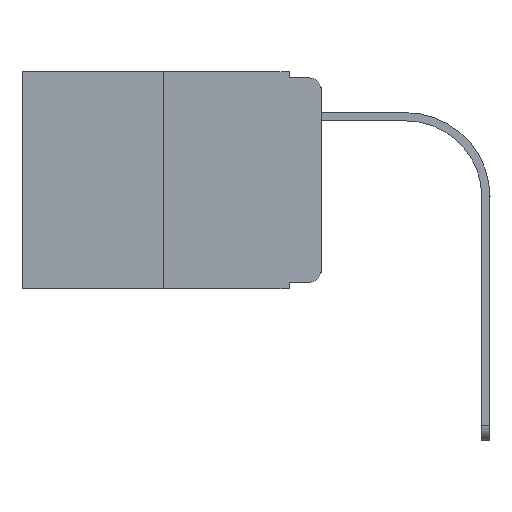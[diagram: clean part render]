
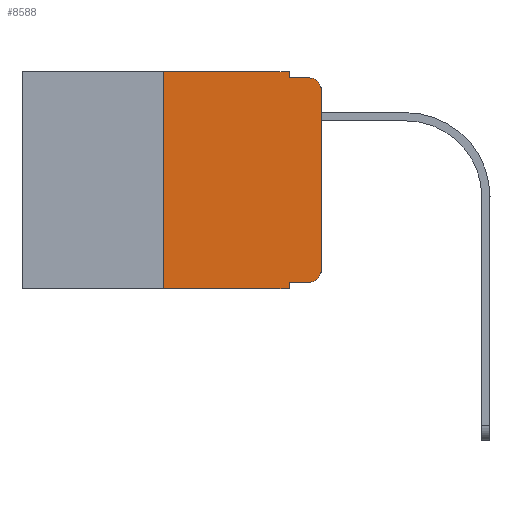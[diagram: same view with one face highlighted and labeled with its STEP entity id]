
A CAD part, left-side view. The second image highlights one B-rep face of the part: STEP entity #8588.
In plain terms, the highlighted planar face has unit normal (-1, 0, 0).
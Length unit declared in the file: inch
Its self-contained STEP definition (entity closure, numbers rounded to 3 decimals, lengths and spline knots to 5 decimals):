
#32 = EDGE_CURVE ( 'NONE', #20131, #15028, #4208, .T. ) ;
#145 = LINE ( 'NONE', #9639, #3905 ) ;
#783 = CARTESIAN_POINT ( 'NONE',  ( 0., 0.02, -0.01 ) ) ;
#1248 = DIRECTION ( 'NONE',  ( 0., 0., -1. ) ) ;
#1324 = VECTOR ( 'NONE', #1902, 39.37008 ) ;
#1642 = PLANE ( 'NONE',  #5877 ) ;
#1818 = CARTESIAN_POINT ( 'NONE',  ( 0., 0.02, -0.333 ) ) ;
#1884 = DIRECTION ( 'NONE',  ( 0., 0., -1. ) ) ;
#1897 = LINE ( 'NONE', #18355, #7198 ) ;
#1902 = DIRECTION ( 'NONE',  ( 0., 0., 1. ) ) ;
#2768 = CARTESIAN_POINT ( 'NONE',  ( 0., 0.051, -0.333 ) ) ;
#3118 = CARTESIAN_POINT ( 'NONE',  ( 0., 0.25, 0. ) ) ;
#3165 = CARTESIAN_POINT ( 'NONE',  ( 0., 0.473, 0. ) ) ;
#3492 = ORIENTED_EDGE ( 'NONE', *, *, #32, .T. ) ;
#3603 = LINE ( 'NONE', #16750, #19665 ) ;
#3665 = CARTESIAN_POINT ( 'NONE',  ( 0., 0., -0.313 ) ) ;
#3905 = VECTOR ( 'NONE', #15010, 39.37008 ) ;
#3970 = EDGE_CURVE ( 'NONE', #7734, #20131, #19240, .T. ) ;
#4208 = LINE ( 'NONE', #7737, #1324 ) ;
#4357 = EDGE_CURVE ( 'NONE', #5290, #7330, #145, .T. ) ;
#4415 = ORIENTED_EDGE ( 'NONE', *, *, #20327, .F. ) ;
#4425 = DIRECTION ( 'NONE',  ( -1., 0., 0. ) ) ;
#4927 = ORIENTED_EDGE ( 'NONE', *, *, #7107, .F. ) ;
#5028 = CIRCLE ( 'NONE', #9308, 0.02 ) ;
#5290 = VERTEX_POINT ( 'NONE', #15312 ) ;
#5820 = DIRECTION ( 'NONE',  ( 0., 0., -1. ) ) ;
#5877 = AXIS2_PLACEMENT_3D ( 'NONE', #16633, #24042, #7369 ) ;
#6357 = EDGE_CURVE ( 'NONE', #15028, #13098, #5028, .T. ) ;
#6481 = ORIENTED_EDGE ( 'NONE', *, *, #20746, .T. ) ;
#6752 = DIRECTION ( 'NONE',  ( 0., 0., 1. ) ) ;
#6993 = CARTESIAN_POINT ( 'NONE',  ( 0., 0.25, 0. ) ) ;
#7107 = EDGE_CURVE ( 'NONE', #20869, #7348, #23554, .T. ) ;
#7198 = VECTOR ( 'NONE', #14710, 39.37008 ) ;
#7330 = VERTEX_POINT ( 'NONE', #16513 ) ;
#7348 = VERTEX_POINT ( 'NONE', #6993 ) ;
#7369 = DIRECTION ( 'NONE',  ( 0., 0., -1. ) ) ;
#7404 = CARTESIAN_POINT ( 'NONE',  ( 0., 0.051, 0. ) ) ;
#7550 = CARTESIAN_POINT ( 'NONE',  ( 0., 0., -0.03 ) ) ;
#7734 = VERTEX_POINT ( 'NONE', #1818 ) ;
#7737 = CARTESIAN_POINT ( 'NONE',  ( 0., 0., 0. ) ) ;
#8588 = ADVANCED_FACE ( 'NONE', ( #21992 ), #1642, .F. ) ;
#8758 = LINE ( 'NONE', #23593, #9509 ) ;
#9102 = VERTEX_POINT ( 'NONE', #22542 ) ;
#9140 = AXIS2_PLACEMENT_3D ( 'NONE', #10508, #4425, #1248 ) ;
#9308 = AXIS2_PLACEMENT_3D ( 'NONE', #16801, #20344, #5820 ) ;
#9509 = VECTOR ( 'NONE', #10824, 39.37008 ) ;
#9639 = CARTESIAN_POINT ( 'NONE',  ( 0., 0.051, 0. ) ) ;
#10508 = CARTESIAN_POINT ( 'NONE',  ( 0., 0.02, -0.313 ) ) ;
#10824 = DIRECTION ( 'NONE',  ( 0., -1., 0. ) ) ;
#11146 = CARTESIAN_POINT ( 'NONE',  ( 0., 0.25, -0.343 ) ) ;
#11247 = ORIENTED_EDGE ( 'NONE', *, *, #22212, .T. ) ;
#11293 = VECTOR ( 'NONE', #12427, 39.37008 ) ;
#11634 = EDGE_CURVE ( 'NONE', #20529, #9102, #3603, .T. ) ;
#12427 = DIRECTION ( 'NONE',  ( 0., -1., 0. ) ) ;
#12439 = VECTOR ( 'NONE', #6752, 39.37008 ) ;
#12999 = VECTOR ( 'NONE', #19696, 39.37008 ) ;
#13098 = VERTEX_POINT ( 'NONE', #783 ) ;
#13335 = ORIENTED_EDGE ( 'NONE', *, *, #17640, .F. ) ;
#14231 = ORIENTED_EDGE ( 'NONE', *, *, #6357, .T. ) ;
#14266 = ORIENTED_EDGE ( 'NONE', *, *, #11634, .F. ) ;
#14710 = DIRECTION ( 'NONE',  ( 0., -1., 0. ) ) ;
#15010 = DIRECTION ( 'NONE',  ( 0., 0., -1. ) ) ;
#15028 = VERTEX_POINT ( 'NONE', #7550 ) ;
#15312 = CARTESIAN_POINT ( 'NONE',  ( 0., 0.051, -0.333 ) ) ;
#16103 = EDGE_LOOP ( 'NONE', ( #3492, #14231, #4415, #14266, #13335, #4927, #11247, #18638, #6481, #19538 ) ) ;
#16513 = CARTESIAN_POINT ( 'NONE',  ( 0., 0.051, -0.343 ) ) ;
#16633 = CARTESIAN_POINT ( 'NONE',  ( 0., 0.473, 0. ) ) ;
#16750 = CARTESIAN_POINT ( 'NONE',  ( 0., 0.051, 0. ) ) ;
#16801 = CARTESIAN_POINT ( 'NONE',  ( 0., 0.02, -0.03 ) ) ;
#17640 = EDGE_CURVE ( 'NONE', #7348, #20529, #23366, .T. ) ;
#18355 = CARTESIAN_POINT ( 'NONE',  ( 0., 0.473, -0.343 ) ) ;
#18638 = ORIENTED_EDGE ( 'NONE', *, *, #4357, .F. ) ;
#19240 = CIRCLE ( 'NONE', #9140, 0.02 ) ;
#19538 = ORIENTED_EDGE ( 'NONE', *, *, #3970, .T. ) ;
#19665 = VECTOR ( 'NONE', #1884, 39.37008 ) ;
#19696 = DIRECTION ( 'NONE',  ( 0., -1., 0. ) ) ;
#20131 = VERTEX_POINT ( 'NONE', #3665 ) ;
#20327 = EDGE_CURVE ( 'NONE', #9102, #13098, #8758, .T. ) ;
#20344 = DIRECTION ( 'NONE',  ( -1., 0., 0. ) ) ;
#20529 = VERTEX_POINT ( 'NONE', #7404 ) ;
#20746 = EDGE_CURVE ( 'NONE', #5290, #7734, #21525, .T. ) ;
#20869 = VERTEX_POINT ( 'NONE', #11146 ) ;
#21525 = LINE ( 'NONE', #2768, #12999 ) ;
#21992 = FACE_OUTER_BOUND ( 'NONE', #16103, .T. ) ;
#22212 = EDGE_CURVE ( 'NONE', #20869, #7330, #1897, .T. ) ;
#22542 = CARTESIAN_POINT ( 'NONE',  ( 0., 0.051, -0.01 ) ) ;
#23366 = LINE ( 'NONE', #3165, #11293 ) ;
#23554 = LINE ( 'NONE', #3118, #12439 ) ;
#23593 = CARTESIAN_POINT ( 'NONE',  ( 0., 0.051, -0.01 ) ) ;
#24042 = DIRECTION ( 'NONE',  ( 1., 0., 0. ) ) ;
